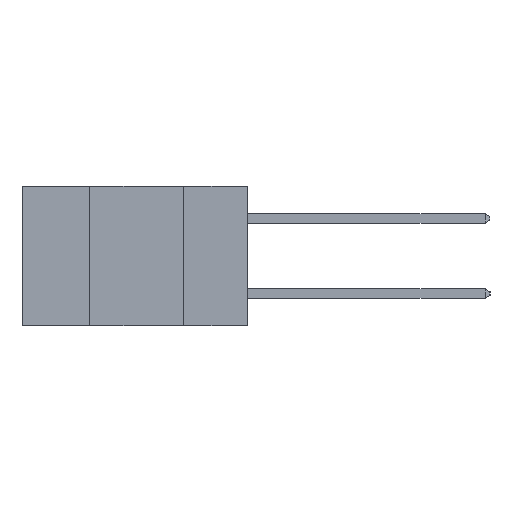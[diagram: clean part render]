
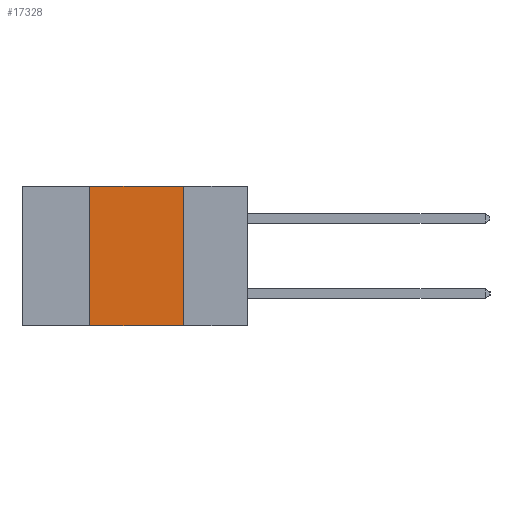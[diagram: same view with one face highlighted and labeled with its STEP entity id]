
A CAD part, left-side view. The second image highlights one B-rep face of the part: STEP entity #17328.
In plain terms, the highlighted planar face has unit normal (-1, 0, 0).
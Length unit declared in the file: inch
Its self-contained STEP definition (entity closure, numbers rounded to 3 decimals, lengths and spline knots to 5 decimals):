
#1101 = CARTESIAN_POINT ( 'NONE',  ( 0., 0.42, 0. ) ) ;
#1223 = CARTESIAN_POINT ( 'NONE',  ( 0., 0.42, -0.37 ) ) ;
#1308 = EDGE_CURVE ( 'NONE', #11424, #8050, #14292, .T. ) ;
#2194 = VECTOR ( 'NONE', #3603, 39.37008 ) ;
#2368 = ORIENTED_EDGE ( 'NONE', *, *, #12569, .F. ) ;
#2425 = EDGE_CURVE ( 'NONE', #16742, #8050, #11017, .T. ) ;
#2637 = CARTESIAN_POINT ( 'NONE',  ( 0., 0.6, 0. ) ) ;
#2768 = VERTEX_POINT ( 'NONE', #1101 ) ;
#3296 = CARTESIAN_POINT ( 'NONE',  ( 0., 0.6, -0.37 ) ) ;
#3378 = VECTOR ( 'NONE', #10703, 39.37008 ) ;
#3603 = DIRECTION ( 'NONE',  ( 0., 0., -1. ) ) ;
#4206 = DIRECTION ( 'NONE',  ( 1., 0., 0. ) ) ;
#6000 = EDGE_CURVE ( 'NONE', #16742, #2768, #9245, .T. ) ;
#8050 = VERTEX_POINT ( 'NONE', #8999 ) ;
#8763 = VECTOR ( 'NONE', #16326, 39.37008 ) ;
#8999 = CARTESIAN_POINT ( 'NONE',  ( 0., 0.17, -0.37 ) ) ;
#9210 = AXIS2_PLACEMENT_3D ( 'NONE', #2637, #4206, #14749 ) ;
#9245 = LINE ( 'NONE', #15935, #8763 ) ;
#10503 = LINE ( 'NONE', #13609, #18352 ) ;
#10703 = DIRECTION ( 'NONE',  ( 0., -1., 0. ) ) ;
#10995 = CARTESIAN_POINT ( 'NONE',  ( 0., 0.17, 0. ) ) ;
#11017 = LINE ( 'NONE', #3296, #3378 ) ;
#11410 = EDGE_LOOP ( 'NONE', ( #11446, #2368, #13977, #17440 ) ) ;
#11424 = VERTEX_POINT ( 'NONE', #10995 ) ;
#11446 = ORIENTED_EDGE ( 'NONE', *, *, #1308, .F. ) ;
#11765 = PLANE ( 'NONE',  #9210 ) ;
#12569 = EDGE_CURVE ( 'NONE', #2768, #11424, #10503, .T. ) ;
#13273 = CARTESIAN_POINT ( 'NONE',  ( 0., 0.17, -0.37 ) ) ;
#13609 = CARTESIAN_POINT ( 'NONE',  ( 0., 0.6, 0. ) ) ;
#13977 = ORIENTED_EDGE ( 'NONE', *, *, #6000, .F. ) ;
#14292 = LINE ( 'NONE', #13273, #2194 ) ;
#14749 = DIRECTION ( 'NONE',  ( 0., 0., -1. ) ) ;
#15115 = DIRECTION ( 'NONE',  ( 0., -1., 0. ) ) ;
#15935 = CARTESIAN_POINT ( 'NONE',  ( 0., 0.42, -0.37 ) ) ;
#16326 = DIRECTION ( 'NONE',  ( 0., 0., 1. ) ) ;
#16742 = VERTEX_POINT ( 'NONE', #1223 ) ;
#17328 = ADVANCED_FACE ( 'NONE', ( #19332 ), #11765, .F. ) ;
#17440 = ORIENTED_EDGE ( 'NONE', *, *, #2425, .T. ) ;
#18352 = VECTOR ( 'NONE', #15115, 39.37008 ) ;
#19332 = FACE_OUTER_BOUND ( 'NONE', #11410, .T. ) ;
